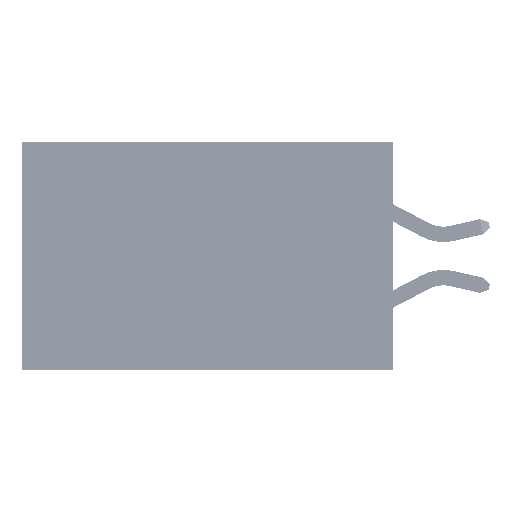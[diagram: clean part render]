
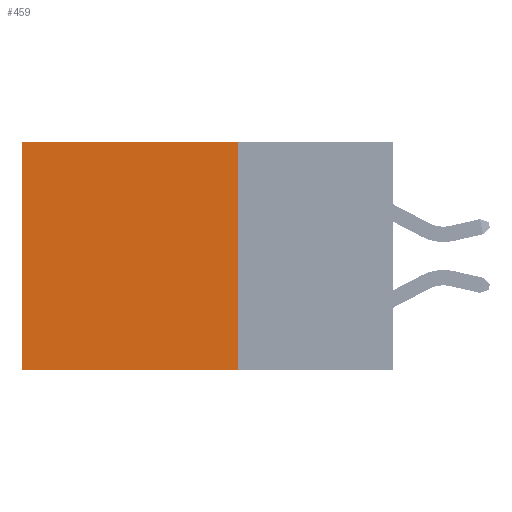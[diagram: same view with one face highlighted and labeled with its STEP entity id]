
A CAD part, left-side view. The second image highlights one B-rep face of the part: STEP entity #459.
In plain terms, the highlighted planar face has unit normal (-1, 0, 0).
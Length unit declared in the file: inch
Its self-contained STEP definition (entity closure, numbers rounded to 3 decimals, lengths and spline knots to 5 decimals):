
#459 = ADVANCED_FACE ( 'NONE', ( #36151 ), #44505, .F. ) ;
#620 = LINE ( 'NONE', #2179, #37896 ) ;
#1869 = ORIENTED_EDGE ( 'NONE', *, *, #35816, .T. ) ;
#2179 = CARTESIAN_POINT ( 'NONE',  ( 0.2875, 0.25, 0. ) ) ;
#3571 = EDGE_LOOP ( 'NONE', ( #22445, #14957, #38533, #1869 ) ) ;
#4528 = LINE ( 'NONE', #34828, #16421 ) ;
#4553 = LINE ( 'NONE', #21629, #16439 ) ;
#9006 = LINE ( 'NONE', #42128, #26494 ) ;
#9795 = DIRECTION ( 'NONE',  ( 0., 0., -1. ) ) ;
#10871 = DIRECTION ( 'NONE',  ( 0., 1., 0. ) ) ;
#14957 = ORIENTED_EDGE ( 'NONE', *, *, #44700, .F. ) ;
#15164 = CARTESIAN_POINT ( 'NONE',  ( 0.2875, 0.25, 0. ) ) ;
#15872 = VERTEX_POINT ( 'NONE', #43103 ) ;
#16421 = VECTOR ( 'NONE', #34213, 39.37008 ) ;
#16439 = VECTOR ( 'NONE', #10871, 39.37008 ) ;
#19274 = VERTEX_POINT ( 'NONE', #44353 ) ;
#21629 = CARTESIAN_POINT ( 'NONE',  ( 0.2875, 0.25, -0.37 ) ) ;
#22445 = ORIENTED_EDGE ( 'NONE', *, *, #25424, .T. ) ;
#25424 = EDGE_CURVE ( 'NONE', #15872, #32060, #4528, .T. ) ;
#26494 = VECTOR ( 'NONE', #9795, 39.37008 ) ;
#27660 = DIRECTION ( 'NONE',  ( 0., 0., -1. ) ) ;
#27695 = VERTEX_POINT ( 'NONE', #15164 ) ;
#30664 = EDGE_CURVE ( 'NONE', #27695, #19274, #9006, .T. ) ;
#31804 = CARTESIAN_POINT ( 'NONE',  ( 0.2875, 0.6, -0.37 ) ) ;
#32060 = VERTEX_POINT ( 'NONE', #31804 ) ;
#33824 = CARTESIAN_POINT ( 'NONE',  ( 0.2875, 0.25, 0. ) ) ;
#34213 = DIRECTION ( 'NONE',  ( 0., 0., -1. ) ) ;
#34776 = DIRECTION ( 'NONE',  ( 1., 0., 0. ) ) ;
#34828 = CARTESIAN_POINT ( 'NONE',  ( 0.2875, 0.6, 0. ) ) ;
#35816 = EDGE_CURVE ( 'NONE', #27695, #15872, #620, .T. ) ;
#36151 = FACE_OUTER_BOUND ( 'NONE', #3571, .T. ) ;
#37896 = VECTOR ( 'NONE', #41610, 39.37008 ) ;
#38533 = ORIENTED_EDGE ( 'NONE', *, *, #30664, .F. ) ;
#41610 = DIRECTION ( 'NONE',  ( 0., 1., 0. ) ) ;
#41800 = AXIS2_PLACEMENT_3D ( 'NONE', #33824, #34776, #27660 ) ;
#42128 = CARTESIAN_POINT ( 'NONE',  ( 0.2875, 0.25, 0. ) ) ;
#43103 = CARTESIAN_POINT ( 'NONE',  ( 0.2875, 0.6, 0. ) ) ;
#44353 = CARTESIAN_POINT ( 'NONE',  ( 0.2875, 0.25, -0.37 ) ) ;
#44505 = PLANE ( 'NONE',  #41800 ) ;
#44700 = EDGE_CURVE ( 'NONE', #19274, #32060, #4553, .T. ) ;
